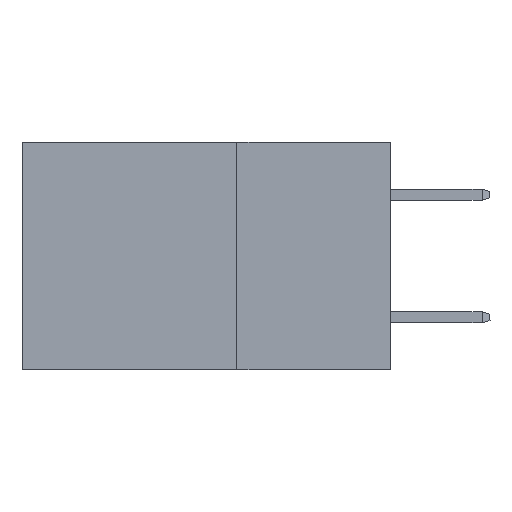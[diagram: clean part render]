
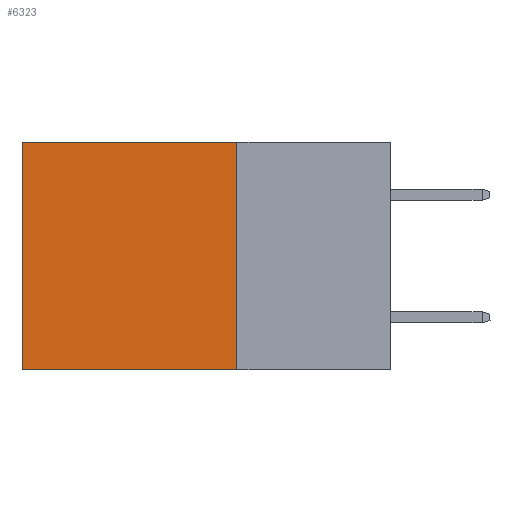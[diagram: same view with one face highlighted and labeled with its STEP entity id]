
A CAD part, left-side view. The second image highlights one B-rep face of the part: STEP entity #6323.
In plain terms, the highlighted planar face has unit normal (-1, 0, 0).
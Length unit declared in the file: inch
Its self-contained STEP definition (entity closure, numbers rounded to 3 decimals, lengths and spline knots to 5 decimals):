
#426 = DIRECTION ( 'NONE',  ( 0., 0., -1. ) ) ;
#525 = DIRECTION ( 'NONE',  ( 0., 0., -1. ) ) ;
#636 = FACE_OUTER_BOUND ( 'NONE', #8842, .T. ) ;
#672 = EDGE_CURVE ( 'NONE', #9721, #10716, #5058, .T. ) ;
#776 = AXIS2_PLACEMENT_3D ( 'NONE', #6402, #2311, #8907 ) ;
#841 = EDGE_CURVE ( 'NONE', #6718, #9721, #5316, .T. ) ;
#1344 = LINE ( 'NONE', #2809, #4025 ) ;
#1837 = CARTESIAN_POINT ( 'NONE',  ( 0.2875, 0.6, 0. ) ) ;
#1928 = VERTEX_POINT ( 'NONE', #1837 ) ;
#2311 = DIRECTION ( 'NONE',  ( 1., 0., 0. ) ) ;
#2809 = CARTESIAN_POINT ( 'NONE',  ( 0.2875, 0.6, 0. ) ) ;
#3708 = DIRECTION ( 'NONE',  ( 0., 1., 0. ) ) ;
#3932 = PLANE ( 'NONE',  #776 ) ;
#4025 = VECTOR ( 'NONE', #525, 39.37008 ) ;
#4563 = CARTESIAN_POINT ( 'NONE',  ( 0.2875, 0.25, 0. ) ) ;
#4600 = CARTESIAN_POINT ( 'NONE',  ( 0.2875, 0.25, -0.37 ) ) ;
#4968 = EDGE_CURVE ( 'NONE', #1928, #10716, #1344, .T. ) ;
#5058 = LINE ( 'NONE', #7600, #5816 ) ;
#5316 = LINE ( 'NONE', #8642, #8601 ) ;
#5587 = ORIENTED_EDGE ( 'NONE', *, *, #672, .F. ) ;
#5816 = VECTOR ( 'NONE', #10075, 39.37008 ) ;
#6175 = LINE ( 'NONE', #4563, #7412 ) ;
#6323 = ADVANCED_FACE ( 'NONE', ( #636 ), #3932, .F. ) ;
#6402 = CARTESIAN_POINT ( 'NONE',  ( 0.2875, 0.25, 0. ) ) ;
#6718 = VERTEX_POINT ( 'NONE', #10656 ) ;
#7412 = VECTOR ( 'NONE', #3708, 39.37008 ) ;
#7424 = CARTESIAN_POINT ( 'NONE',  ( 0.2875, 0.6, -0.37 ) ) ;
#7600 = CARTESIAN_POINT ( 'NONE',  ( 0.2875, 0.25, -0.37 ) ) ;
#7845 = EDGE_CURVE ( 'NONE', #6718, #1928, #6175, .T. ) ;
#8601 = VECTOR ( 'NONE', #426, 39.37008 ) ;
#8642 = CARTESIAN_POINT ( 'NONE',  ( 0.2875, 0.25, 0. ) ) ;
#8823 = ORIENTED_EDGE ( 'NONE', *, *, #841, .F. ) ;
#8842 = EDGE_LOOP ( 'NONE', ( #9166, #5587, #8823, #9865 ) ) ;
#8907 = DIRECTION ( 'NONE',  ( 0., 0., -1. ) ) ;
#9166 = ORIENTED_EDGE ( 'NONE', *, *, #4968, .T. ) ;
#9721 = VERTEX_POINT ( 'NONE', #4600 ) ;
#9865 = ORIENTED_EDGE ( 'NONE', *, *, #7845, .T. ) ;
#10075 = DIRECTION ( 'NONE',  ( 0., 1., 0. ) ) ;
#10656 = CARTESIAN_POINT ( 'NONE',  ( 0.2875, 0.25, 0. ) ) ;
#10716 = VERTEX_POINT ( 'NONE', #7424 ) ;
